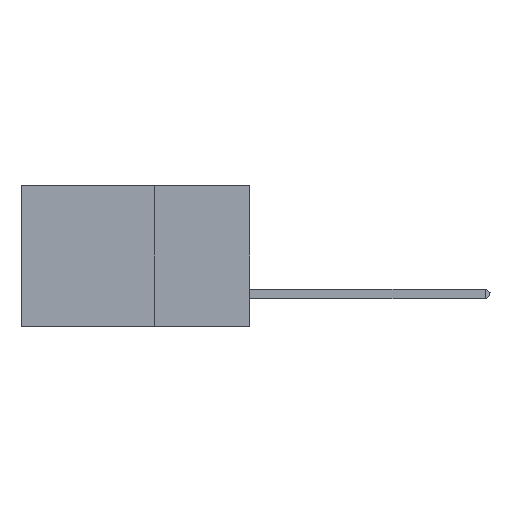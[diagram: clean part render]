
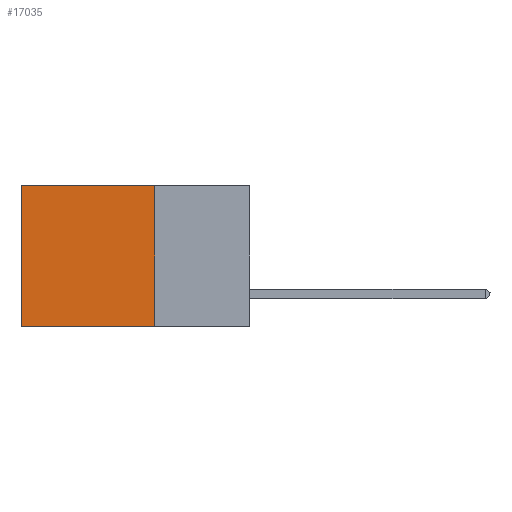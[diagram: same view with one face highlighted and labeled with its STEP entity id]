
A CAD part, left-side view. The second image highlights one B-rep face of the part: STEP entity #17035.
In plain terms, the highlighted planar face has unit normal (-1, 0, 0).
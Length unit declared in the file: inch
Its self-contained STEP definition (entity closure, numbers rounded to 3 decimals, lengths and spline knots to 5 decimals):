
#440 = LINE ( 'NONE', #5099, #9820 ) ;
#541 = ORIENTED_EDGE ( 'NONE', *, *, #3564, .F. ) ;
#799 = VERTEX_POINT ( 'NONE', #10856 ) ;
#1051 = LINE ( 'NONE', #12992, #6039 ) ;
#1243 = CARTESIAN_POINT ( 'NONE',  ( 0.2875, 0.6, 0. ) ) ;
#1399 = CARTESIAN_POINT ( 'NONE',  ( 0.2875, 0.25, 0. ) ) ;
#1675 = CARTESIAN_POINT ( 'NONE',  ( 0.2875, 0.25, -0.37 ) ) ;
#2437 = VERTEX_POINT ( 'NONE', #1243 ) ;
#2672 = PLANE ( 'NONE',  #13784 ) ;
#3564 = EDGE_CURVE ( 'NONE', #799, #5408, #3953, .T. ) ;
#3953 = LINE ( 'NONE', #1399, #10912 ) ;
#4581 = EDGE_CURVE ( 'NONE', #2437, #9040, #8465, .T. ) ;
#4784 = DIRECTION ( 'NONE',  ( 0., 0., -1. ) ) ;
#5099 = CARTESIAN_POINT ( 'NONE',  ( 0.2875, 0.25, 0. ) ) ;
#5408 = VERTEX_POINT ( 'NONE', #1675 ) ;
#5652 = DIRECTION ( 'NONE',  ( 0., 0., -1. ) ) ;
#5700 = EDGE_CURVE ( 'NONE', #5408, #9040, #1051, .T. ) ;
#6039 = VECTOR ( 'NONE', #14158, 39.37008 ) ;
#6687 = CARTESIAN_POINT ( 'NONE',  ( 0.2875, 0.25, 0. ) ) ;
#7158 = FACE_OUTER_BOUND ( 'NONE', #9308, .T. ) ;
#8465 = LINE ( 'NONE', #8903, #8915 ) ;
#8903 = CARTESIAN_POINT ( 'NONE',  ( 0.2875, 0.6, 0. ) ) ;
#8915 = VECTOR ( 'NONE', #4784, 39.37008 ) ;
#9040 = VERTEX_POINT ( 'NONE', #14489 ) ;
#9308 = EDGE_LOOP ( 'NONE', ( #11767, #14237, #541, #9772 ) ) ;
#9772 = ORIENTED_EDGE ( 'NONE', *, *, #15521, .T. ) ;
#9820 = VECTOR ( 'NONE', #14851, 39.37008 ) ;
#10856 = CARTESIAN_POINT ( 'NONE',  ( 0.2875, 0.25, 0. ) ) ;
#10912 = VECTOR ( 'NONE', #5652, 39.37008 ) ;
#11767 = ORIENTED_EDGE ( 'NONE', *, *, #4581, .T. ) ;
#12416 = DIRECTION ( 'NONE',  ( 0., 0., -1. ) ) ;
#12992 = CARTESIAN_POINT ( 'NONE',  ( 0.2875, 0.25, -0.37 ) ) ;
#13784 = AXIS2_PLACEMENT_3D ( 'NONE', #6687, #16628, #12416 ) ;
#14158 = DIRECTION ( 'NONE',  ( 0., 1., 0. ) ) ;
#14237 = ORIENTED_EDGE ( 'NONE', *, *, #5700, .F. ) ;
#14489 = CARTESIAN_POINT ( 'NONE',  ( 0.2875, 0.6, -0.37 ) ) ;
#14851 = DIRECTION ( 'NONE',  ( 0., 1., 0. ) ) ;
#15521 = EDGE_CURVE ( 'NONE', #799, #2437, #440, .T. ) ;
#16628 = DIRECTION ( 'NONE',  ( 1., 0., 0. ) ) ;
#17035 = ADVANCED_FACE ( 'NONE', ( #7158 ), #2672, .F. ) ;
